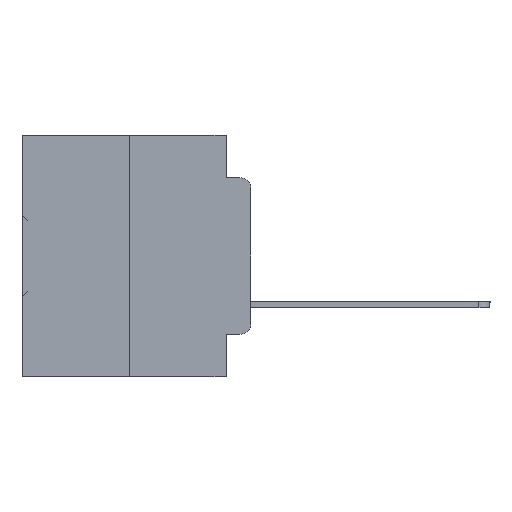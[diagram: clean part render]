
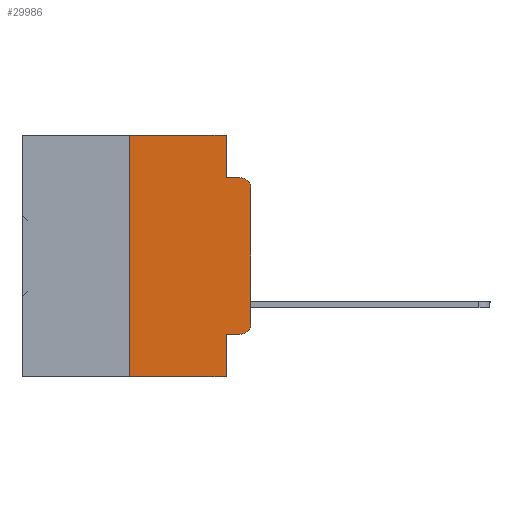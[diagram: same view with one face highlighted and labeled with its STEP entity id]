
A CAD part, left-side view. The second image highlights one B-rep face of the part: STEP entity #29986.
In plain terms, the highlighted planar face has unit normal (-1, 0, 0).
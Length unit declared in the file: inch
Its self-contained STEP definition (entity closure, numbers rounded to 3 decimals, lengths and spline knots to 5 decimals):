
#358 = DIRECTION ( 'NONE',  ( 0., -1., 0. ) ) ;
#517 = CARTESIAN_POINT ( 'NONE',  ( 0., 0.02, -0.1085 ) ) ;
#1066 = EDGE_CURVE ( 'NONE', #19045, #36335, #9352, .T. ) ;
#1645 = DIRECTION ( 'NONE',  ( 0., 0., -1. ) ) ;
#1759 = AXIS2_PLACEMENT_3D ( 'NONE', #37221, #10945, #13445 ) ;
#2188 = LINE ( 'NONE', #35002, #3895 ) ;
#2443 = CARTESIAN_POINT ( 'NONE',  ( 0., 0.473, -0.5 ) ) ;
#3733 = EDGE_CURVE ( 'NONE', #25787, #30735, #16667, .T. ) ;
#3734 = VECTOR ( 'NONE', #27787, 39.37008 ) ;
#3895 = VECTOR ( 'NONE', #13766, 39.37008 ) ;
#4822 = DIRECTION ( 'NONE',  ( -1., 0., 0. ) ) ;
#5149 = CIRCLE ( 'NONE', #18097, 0.02 ) ;
#5346 = LINE ( 'NONE', #2443, #30552 ) ;
#6962 = EDGE_CURVE ( 'NONE', #24305, #27193, #5149, .T. ) ;
#7527 = DIRECTION ( 'NONE',  ( 0., 0., -1. ) ) ;
#7604 = ORIENTED_EDGE ( 'NONE', *, *, #21597, .T. ) ;
#7758 = VERTEX_POINT ( 'NONE', #21653 ) ;
#8089 = CARTESIAN_POINT ( 'NONE',  ( 0., 0., -0.3915 ) ) ;
#8230 = CARTESIAN_POINT ( 'NONE',  ( 0., 0.051, -0.4115 ) ) ;
#8277 = CARTESIAN_POINT ( 'NONE',  ( 0., 0.02, -0.0885 ) ) ;
#9026 = ORIENTED_EDGE ( 'NONE', *, *, #13821, .F. ) ;
#9352 = LINE ( 'NONE', #12050, #30289 ) ;
#9545 = EDGE_CURVE ( 'NONE', #27193, #28266, #24713, .T. ) ;
#10945 = DIRECTION ( 'NONE',  ( 1., 0., 0. ) ) ;
#12050 = CARTESIAN_POINT ( 'NONE',  ( 0., 0.25, 0. ) ) ;
#12059 = AXIS2_PLACEMENT_3D ( 'NONE', #517, #12287, #1645 ) ;
#12287 = DIRECTION ( 'NONE',  ( -1., 0., 0. ) ) ;
#12760 = CARTESIAN_POINT ( 'NONE',  ( 0., 0.25, -0.5 ) ) ;
#13445 = DIRECTION ( 'NONE',  ( 0., 0., -1. ) ) ;
#13766 = DIRECTION ( 'NONE',  ( 0., 0., -1. ) ) ;
#13768 = CARTESIAN_POINT ( 'NONE',  ( 0., 0.051, -0.0885 ) ) ;
#13821 = EDGE_CURVE ( 'NONE', #26690, #7758, #2188, .T. ) ;
#15116 = ORIENTED_EDGE ( 'NONE', *, *, #9545, .T. ) ;
#15925 = VECTOR ( 'NONE', #7527, 39.37008 ) ;
#16151 = ORIENTED_EDGE ( 'NONE', *, *, #6962, .T. ) ;
#16572 = EDGE_CURVE ( 'NONE', #26690, #24305, #34695, .T. ) ;
#16618 = VECTOR ( 'NONE', #20033, 39.37008 ) ;
#16667 = LINE ( 'NONE', #13768, #20144 ) ;
#16782 = CARTESIAN_POINT ( 'NONE',  ( 0., 0.051, 0. ) ) ;
#18097 = AXIS2_PLACEMENT_3D ( 'NONE', #33603, #4822, #27629 ) ;
#19045 = VERTEX_POINT ( 'NONE', #12760 ) ;
#20033 = DIRECTION ( 'NONE',  ( 0., -1., 0. ) ) ;
#20144 = VECTOR ( 'NONE', #25567, 39.37008 ) ;
#20203 = EDGE_CURVE ( 'NONE', #19045, #7758, #5346, .T. ) ;
#21158 = DIRECTION ( 'NONE',  ( 0., 0., 1. ) ) ;
#21597 = EDGE_CURVE ( 'NONE', #28266, #30735, #37967, .T. ) ;
#21653 = CARTESIAN_POINT ( 'NONE',  ( 0., 0.051, -0.5 ) ) ;
#22207 = CARTESIAN_POINT ( 'NONE',  ( 0., 0.051, -0.0885 ) ) ;
#22940 = VERTEX_POINT ( 'NONE', #33579 ) ;
#24305 = VERTEX_POINT ( 'NONE', #35146 ) ;
#24713 = LINE ( 'NONE', #33387, #3734 ) ;
#25027 = ORIENTED_EDGE ( 'NONE', *, *, #1066, .F. ) ;
#25309 = LINE ( 'NONE', #16782, #15925 ) ;
#25567 = DIRECTION ( 'NONE',  ( 0., -1., 0. ) ) ;
#25787 = VERTEX_POINT ( 'NONE', #22207 ) ;
#26690 = VERTEX_POINT ( 'NONE', #32064 ) ;
#26825 = CARTESIAN_POINT ( 'NONE',  ( 0., 0.473, 0. ) ) ;
#27193 = VERTEX_POINT ( 'NONE', #8089 ) ;
#27629 = DIRECTION ( 'NONE',  ( 0., 0., -1. ) ) ;
#27787 = DIRECTION ( 'NONE',  ( 0., 0., 1. ) ) ;
#28139 = PLANE ( 'NONE',  #1759 ) ;
#28266 = VERTEX_POINT ( 'NONE', #36686 ) ;
#28877 = ORIENTED_EDGE ( 'NONE', *, *, #30829, .F. ) ;
#29083 = DIRECTION ( 'NONE',  ( 0., -1., 0. ) ) ;
#29463 = EDGE_CURVE ( 'NONE', #22940, #25787, #25309, .T. ) ;
#29986 = ADVANCED_FACE ( 'NONE', ( #36836 ), #28139, .F. ) ;
#30289 = VECTOR ( 'NONE', #21158, 39.37008 ) ;
#30552 = VECTOR ( 'NONE', #29083, 39.37008 ) ;
#30735 = VERTEX_POINT ( 'NONE', #8277 ) ;
#30829 = EDGE_CURVE ( 'NONE', #36335, #22940, #32613, .T. ) ;
#32064 = CARTESIAN_POINT ( 'NONE',  ( 0., 0.051, -0.4115 ) ) ;
#32325 = CARTESIAN_POINT ( 'NONE',  ( 0., 0.25, 0. ) ) ;
#32469 = ORIENTED_EDGE ( 'NONE', *, *, #29463, .F. ) ;
#32613 = LINE ( 'NONE', #26825, #34499 ) ;
#33387 = CARTESIAN_POINT ( 'NONE',  ( 0., 0., 0. ) ) ;
#33498 = ORIENTED_EDGE ( 'NONE', *, *, #20203, .T. ) ;
#33579 = CARTESIAN_POINT ( 'NONE',  ( 0., 0.051, 0. ) ) ;
#33603 = CARTESIAN_POINT ( 'NONE',  ( 0., 0.02, -0.3915 ) ) ;
#34499 = VECTOR ( 'NONE', #358, 39.37008 ) ;
#34695 = LINE ( 'NONE', #8230, #16618 ) ;
#35002 = CARTESIAN_POINT ( 'NONE',  ( 0., 0.051, 0. ) ) ;
#35146 = CARTESIAN_POINT ( 'NONE',  ( 0., 0.02, -0.4115 ) ) ;
#36335 = VERTEX_POINT ( 'NONE', #32325 ) ;
#36686 = CARTESIAN_POINT ( 'NONE',  ( 0., 0., -0.1085 ) ) ;
#36836 = FACE_OUTER_BOUND ( 'NONE', #36845, .T. ) ;
#36845 = EDGE_LOOP ( 'NONE', ( #15116, #7604, #36987, #32469, #28877, #25027, #33498, #9026, #37033, #16151 ) ) ;
#36987 = ORIENTED_EDGE ( 'NONE', *, *, #3733, .F. ) ;
#37033 = ORIENTED_EDGE ( 'NONE', *, *, #16572, .T. ) ;
#37221 = CARTESIAN_POINT ( 'NONE',  ( 0., 0.473, 0. ) ) ;
#37967 = CIRCLE ( 'NONE', #12059, 0.02 ) ;
